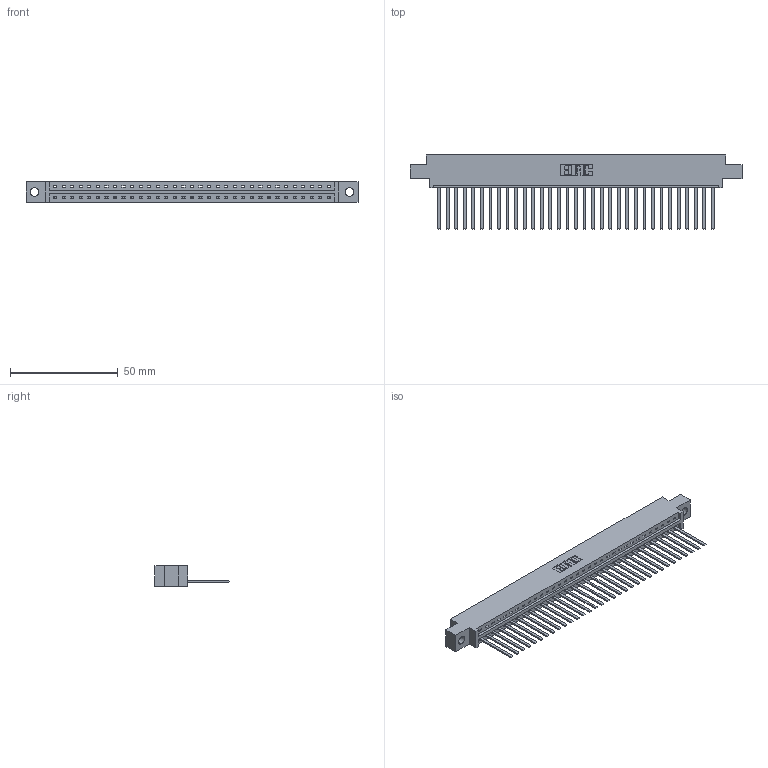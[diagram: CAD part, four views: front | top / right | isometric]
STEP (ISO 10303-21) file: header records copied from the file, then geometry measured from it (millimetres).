
FILE_DESCRIPTION (( 'STEP AP203' ), '1' );
FILE_NAME ('337-033-544-604.STEP', '2019-10-01T11:06:12', ( '' ), ( '' ), 'SwSTEP 2.0', 'SolidWorks 2016', '' );
FILE_SCHEMA (( 'CONFIG_CONTROL_DESIGN' ));
Length unit declared in the file: inch
Products named in the file (3): 337 Part_0.170 Offset - 0.156 Dia-TH; 337-033-544-604; 345-292-001_345-293-144
Assembly tree (34 placements, depth 2):
  337-033-544-604
    337 Part_0.170 Offset - 0.156 Dia-TH
    345-292-001_345-293-144  x33
Bounding box: 153.77 x 34.3 x 9.4 mm (x, y, z)
Volume: 16046.2 mm3; surface area: 17680.3 mm2
Topology: 34 solids, 34 shells, 1966 faces, 5933 edges, 3910 vertices
Faces by surface type: plane 1460, cylinder 506
Entity records: 25645 total; most frequent: CARTESIAN_POINT 4473, ORIENTED_EDGE 4442, DIRECTION 3779, EDGE_CURVE 2221, VECTOR 2097, LINE 2097, VERTEX_POINT 1478, AXIS2_PLACEMENT_3D 841
